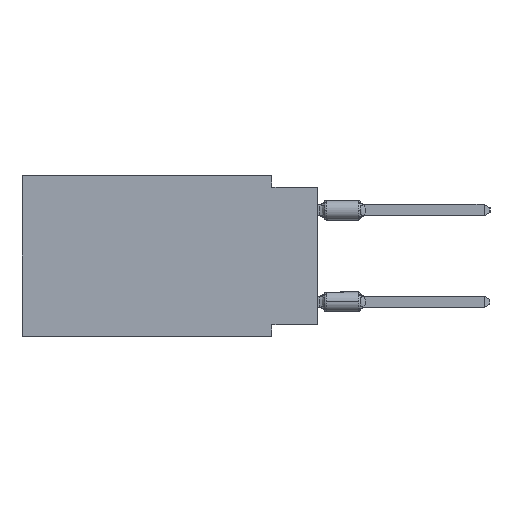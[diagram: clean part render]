
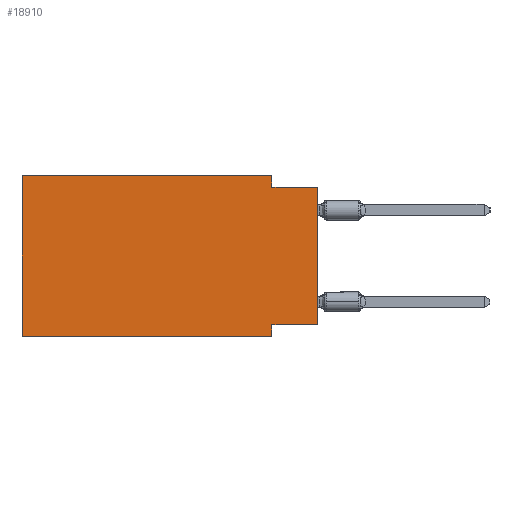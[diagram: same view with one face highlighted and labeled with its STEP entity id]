
A CAD part, left-side view. The second image highlights one B-rep face of the part: STEP entity #18910.
In plain terms, the highlighted planar face has unit normal (-1, 0, 0).
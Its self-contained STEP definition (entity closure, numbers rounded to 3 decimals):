
#456 = DIRECTION ( 'NONE',  ( 0., -1., 0. ) ) ;
#499 = DIRECTION ( 'NONE',  ( 0., -1., 0. ) ) ;
#715 = VERTEX_POINT ( 'NONE', #8238 ) ;
#726 = ORIENTED_EDGE ( 'NONE', *, *, #1386, .F. ) ;
#1314 = DIRECTION ( 'NONE',  ( 0., 0., 1. ) ) ;
#1386 = EDGE_CURVE ( 'NONE', #715, #46024, #48589, .T. ) ;
#2134 = VECTOR ( 'NONE', #50099, 1000. ) ;
#2165 = EDGE_CURVE ( 'NONE', #46024, #20455, #50200, .T. ) ;
#2399 = ORIENTED_EDGE ( 'NONE', *, *, #54427, .F. ) ;
#3724 = EDGE_CURVE ( 'NONE', #41210, #44733, #39420, .T. ) ;
#3802 = DIRECTION ( 'NONE',  ( 0., 0., -1. ) ) ;
#4114 = VERTEX_POINT ( 'NONE', #15486 ) ;
#5474 = ORIENTED_EDGE ( 'NONE', *, *, #10583, .F. ) ;
#5965 = PLANE ( 'NONE',  #55197 ) ;
#8238 = CARTESIAN_POINT ( 'NONE',  ( 0., 16.383, 0. ) ) ;
#9636 = VECTOR ( 'NONE', #456, 1000. ) ;
#10583 = EDGE_CURVE ( 'NONE', #41210, #715, #20905, .T. ) ;
#13888 = ORIENTED_EDGE ( 'NONE', *, *, #19863, .F. ) ;
#15486 = CARTESIAN_POINT ( 'NONE',  ( 0., 0., -0.635 ) ) ;
#15721 = ORIENTED_EDGE ( 'NONE', *, *, #28801, .T. ) ;
#16774 = LINE ( 'NONE', #27151, #51122 ) ;
#17268 = VERTEX_POINT ( 'NONE', #35751 ) ;
#17274 = CARTESIAN_POINT ( 'NONE',  ( 0., 16.383, 0. ) ) ;
#18910 = ADVANCED_FACE ( 'NONE', ( #36100 ), #5965, .F. ) ;
#19785 = CARTESIAN_POINT ( 'NONE',  ( 0., 16.383, 0. ) ) ;
#19863 = EDGE_CURVE ( 'NONE', #20455, #4114, #34996, .T. ) ;
#20455 = VERTEX_POINT ( 'NONE', #53541 ) ;
#20905 = LINE ( 'NONE', #19785, #46429 ) ;
#23072 = CARTESIAN_POINT ( 'NONE',  ( 0., 2.54, -8.89 ) ) ;
#25618 = CARTESIAN_POINT ( 'NONE',  ( 0., 16.383, -8.89 ) ) ;
#26178 = CARTESIAN_POINT ( 'NONE',  ( 0., 0., -0.635 ) ) ;
#27151 = CARTESIAN_POINT ( 'NONE',  ( 0., 0., 0. ) ) ;
#28607 = DIRECTION ( 'NONE',  ( 0., 0., 1. ) ) ;
#28801 = EDGE_CURVE ( 'NONE', #44888, #4114, #16774, .T. ) ;
#29480 = VECTOR ( 'NONE', #3802, 1000. ) ;
#29665 = EDGE_CURVE ( 'NONE', #17268, #44733, #49534, .T. ) ;
#31116 = CARTESIAN_POINT ( 'NONE',  ( 0., 2.54, 0. ) ) ;
#31270 = DIRECTION ( 'NONE',  ( 0., 0., -1. ) ) ;
#31287 = CARTESIAN_POINT ( 'NONE',  ( 0., 0., -8.255 ) ) ;
#34996 = LINE ( 'NONE', #26178, #47399 ) ;
#35258 = DIRECTION ( 'NONE',  ( 0., -1., 0. ) ) ;
#35555 = LINE ( 'NONE', #31287, #55003 ) ;
#35751 = CARTESIAN_POINT ( 'NONE',  ( 0., 2.54, -8.255 ) ) ;
#36100 = FACE_OUTER_BOUND ( 'NONE', #42942, .T. ) ;
#36116 = ORIENTED_EDGE ( 'NONE', *, *, #29665, .F. ) ;
#39131 = CARTESIAN_POINT ( 'NONE',  ( 0., 16.383, -8.89 ) ) ;
#39420 = LINE ( 'NONE', #39131, #9636 ) ;
#40650 = CARTESIAN_POINT ( 'NONE',  ( 0., 16.383, 0. ) ) ;
#41179 = ORIENTED_EDGE ( 'NONE', *, *, #3724, .T. ) ;
#41210 = VERTEX_POINT ( 'NONE', #25618 ) ;
#42759 = CARTESIAN_POINT ( 'NONE',  ( 0., 2.54, 0. ) ) ;
#42942 = EDGE_LOOP ( 'NONE', ( #15721, #13888, #49497, #726, #5474, #41179, #36116, #2399 ) ) ;
#44733 = VERTEX_POINT ( 'NONE', #51581 ) ;
#44888 = VERTEX_POINT ( 'NONE', #45002 ) ;
#45002 = CARTESIAN_POINT ( 'NONE',  ( 0., 0., -8.255 ) ) ;
#46024 = VERTEX_POINT ( 'NONE', #31116 ) ;
#46429 = VECTOR ( 'NONE', #28607, 1000. ) ;
#47399 = VECTOR ( 'NONE', #35258, 1000. ) ;
#48589 = LINE ( 'NONE', #17274, #55864 ) ;
#49497 = ORIENTED_EDGE ( 'NONE', *, *, #2165, .F. ) ;
#49534 = LINE ( 'NONE', #23072, #2134 ) ;
#50099 = DIRECTION ( 'NONE',  ( 0., 0., -1. ) ) ;
#50200 = LINE ( 'NONE', #42759, #29480 ) ;
#51122 = VECTOR ( 'NONE', #1314, 1000. ) ;
#51581 = CARTESIAN_POINT ( 'NONE',  ( 0., 2.54, -8.89 ) ) ;
#52109 = DIRECTION ( 'NONE',  ( 0., 1., 0. ) ) ;
#53477 = DIRECTION ( 'NONE',  ( 1., 0., 0. ) ) ;
#53541 = CARTESIAN_POINT ( 'NONE',  ( 0., 2.54, -0.635 ) ) ;
#54427 = EDGE_CURVE ( 'NONE', #44888, #17268, #35555, .T. ) ;
#55003 = VECTOR ( 'NONE', #52109, 1000. ) ;
#55197 = AXIS2_PLACEMENT_3D ( 'NONE', #40650, #53477, #31270 ) ;
#55864 = VECTOR ( 'NONE', #499, 1000. ) ;
